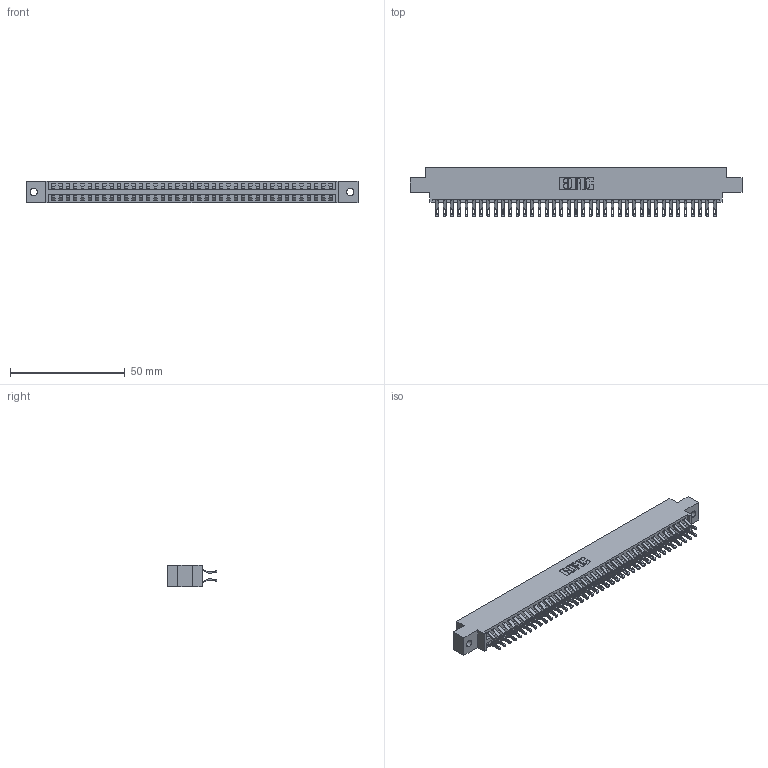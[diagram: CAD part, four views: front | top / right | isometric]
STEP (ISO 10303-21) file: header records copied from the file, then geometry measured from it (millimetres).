
FILE_DESCRIPTION (( 'STEP AP203' ), '1' );
FILE_NAME ('396-078-555-802.STEP', '2018-09-09T17:12:31', ( '' ), ( '' ), 'SwSTEP 2.0', 'SolidWorks 2016', '' );
FILE_SCHEMA (( 'CONFIG_CONTROL_DESIGN' ));
Length unit declared in the file: inch
Products named in the file (3): 345-292-001_555 Tail; 396-078-555-802; 346 Part_0.170 Offset - 0.128 Dia
Assembly tree (79 placements, depth 2):
  396-078-555-802
    346 Part_0.170 Offset - 0.128 Dia
    345-292-001_555 Tail  x78
Bounding box: 144.4 x 21.46 x 9.4 mm (x, y, z)
Volume: 14092.3 mm3; surface area: 20040.6 mm2
Topology: 79 solids, 79 shells, 4650 faces, 14615 edges, 9742 vertices
Faces by surface type: plane 2654, cylinder 1996
Entity records: 26317 total; most frequent: CARTESIAN_POINT 4378, ORIENTED_EDGE 4282, DIRECTION 3877, EDGE_CURVE 2141, LINE 1833, VECTOR 1833, VERTEX_POINT 1426, AXIS2_PLACEMENT_3D 1022
